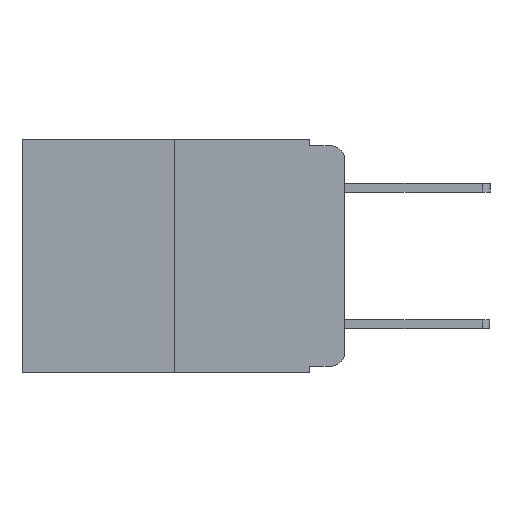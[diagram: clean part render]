
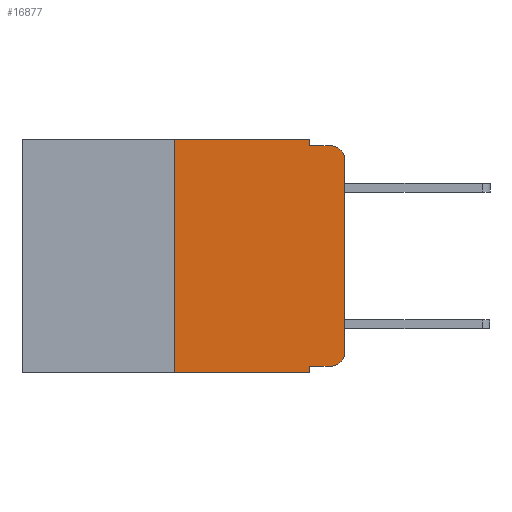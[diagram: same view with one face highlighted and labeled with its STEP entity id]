
A CAD part, left-side view. The second image highlights one B-rep face of the part: STEP entity #16877.
In plain terms, the highlighted planar face has unit normal (-1, 0, 0).
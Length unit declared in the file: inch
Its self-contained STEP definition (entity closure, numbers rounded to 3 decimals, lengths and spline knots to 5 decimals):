
#181 = CARTESIAN_POINT ( 'NONE',  ( 0., 0.02, -0.313 ) ) ;
#188 = ORIENTED_EDGE ( 'NONE', *, *, #11246, .F. ) ;
#422 = VECTOR ( 'NONE', #9994, 39.37008 ) ;
#472 = EDGE_CURVE ( 'NONE', #6923, #17972, #3150, .T. ) ;
#494 = CARTESIAN_POINT ( 'NONE',  ( 0., 0.02, -0.01 ) ) ;
#536 = VECTOR ( 'NONE', #15269, 39.37008 ) ;
#677 = CARTESIAN_POINT ( 'NONE',  ( 0., 0.051, 0. ) ) ;
#696 = DIRECTION ( 'NONE',  ( 0., 0., 1. ) ) ;
#856 = DIRECTION ( 'NONE',  ( 0., 0., -1. ) ) ;
#1072 = ORIENTED_EDGE ( 'NONE', *, *, #9090, .F. ) ;
#1203 = DIRECTION ( 'NONE',  ( 1., 0., 0. ) ) ;
#1535 = EDGE_CURVE ( 'NONE', #9163, #8153, #5222, .T. ) ;
#1844 = DIRECTION ( 'NONE',  ( 0., 0., -1. ) ) ;
#1879 = DIRECTION ( 'NONE',  ( 0., -1., 0. ) ) ;
#1966 = VERTEX_POINT ( 'NONE', #494 ) ;
#2134 = VERTEX_POINT ( 'NONE', #20420 ) ;
#2194 = DIRECTION ( 'NONE',  ( 0., 0., -1. ) ) ;
#2474 = CARTESIAN_POINT ( 'NONE',  ( 0., 0.25, 0. ) ) ;
#3150 = LINE ( 'NONE', #15766, #17242 ) ;
#3175 = CARTESIAN_POINT ( 'NONE',  ( 0., 0., -0.03 ) ) ;
#3643 = VECTOR ( 'NONE', #18622, 39.37008 ) ;
#4335 = EDGE_CURVE ( 'NONE', #6923, #13541, #10631, .T. ) ;
#4337 = VECTOR ( 'NONE', #696, 39.37008 ) ;
#4465 = VERTEX_POINT ( 'NONE', #3175 ) ;
#4986 = CARTESIAN_POINT ( 'NONE',  ( 0., 0.25, 0. ) ) ;
#5062 = CARTESIAN_POINT ( 'NONE',  ( 0., 0., -0.313 ) ) ;
#5222 = LINE ( 'NONE', #677, #20257 ) ;
#5465 = CIRCLE ( 'NONE', #12598, 0.02 ) ;
#5692 = ORIENTED_EDGE ( 'NONE', *, *, #8488, .T. ) ;
#5701 = VECTOR ( 'NONE', #1879, 39.37008 ) ;
#5923 = CARTESIAN_POINT ( 'NONE',  ( 0., 0.051, -0.01 ) ) ;
#6575 = EDGE_LOOP ( 'NONE', ( #7761, #5692, #1072, #21569, #188, #17412, #22151, #22701, #7277, #10739 ) ) ;
#6589 = AXIS2_PLACEMENT_3D ( 'NONE', #12545, #1203, #14337 ) ;
#6639 = CIRCLE ( 'NONE', #22600, 0.02 ) ;
#6923 = VERTEX_POINT ( 'NONE', #18823 ) ;
#7011 = PLANE ( 'NONE',  #6589 ) ;
#7151 = EDGE_CURVE ( 'NONE', #10072, #4465, #23081, .T. ) ;
#7277 = ORIENTED_EDGE ( 'NONE', *, *, #9671, .T. ) ;
#7761 = ORIENTED_EDGE ( 'NONE', *, *, #7151, .T. ) ;
#7845 = CARTESIAN_POINT ( 'NONE',  ( 0., 0.051, -0.333 ) ) ;
#8153 = VERTEX_POINT ( 'NONE', #12173 ) ;
#8488 = EDGE_CURVE ( 'NONE', #4465, #1966, #6639, .T. ) ;
#8598 = EDGE_CURVE ( 'NONE', #2134, #10072, #5465, .T. ) ;
#9090 = EDGE_CURVE ( 'NONE', #8153, #1966, #13510, .T. ) ;
#9163 = VERTEX_POINT ( 'NONE', #17074 ) ;
#9378 = DIRECTION ( 'NONE',  ( 0., -1., 0. ) ) ;
#9511 = CARTESIAN_POINT ( 'NONE',  ( 0., 0.051, -0.333 ) ) ;
#9671 = EDGE_CURVE ( 'NONE', #14532, #2134, #15436, .T. ) ;
#9994 = DIRECTION ( 'NONE',  ( 0., 0., 1. ) ) ;
#10072 = VERTEX_POINT ( 'NONE', #5062 ) ;
#10631 = LINE ( 'NONE', #2474, #422 ) ;
#10739 = ORIENTED_EDGE ( 'NONE', *, *, #8598, .T. ) ;
#11246 = EDGE_CURVE ( 'NONE', #13541, #9163, #15990, .T. ) ;
#12173 = CARTESIAN_POINT ( 'NONE',  ( 0., 0.051, -0.01 ) ) ;
#12250 = CARTESIAN_POINT ( 'NONE',  ( 0., 0., 0. ) ) ;
#12545 = CARTESIAN_POINT ( 'NONE',  ( 0., 0.473, 0. ) ) ;
#12598 = AXIS2_PLACEMENT_3D ( 'NONE', #181, #13422, #2194 ) ;
#13100 = DIRECTION ( 'NONE',  ( -1., 0., 0. ) ) ;
#13422 = DIRECTION ( 'NONE',  ( -1., 0., 0. ) ) ;
#13458 = FACE_OUTER_BOUND ( 'NONE', #6575, .T. ) ;
#13510 = LINE ( 'NONE', #5923, #3643 ) ;
#13541 = VERTEX_POINT ( 'NONE', #4986 ) ;
#14337 = DIRECTION ( 'NONE',  ( 0., 0., -1. ) ) ;
#14532 = VERTEX_POINT ( 'NONE', #7845 ) ;
#15258 = EDGE_CURVE ( 'NONE', #14532, #17972, #20799, .T. ) ;
#15269 = DIRECTION ( 'NONE',  ( 0., 0., -1. ) ) ;
#15436 = LINE ( 'NONE', #9511, #5701 ) ;
#15766 = CARTESIAN_POINT ( 'NONE',  ( 0., 0.473, -0.343 ) ) ;
#15990 = LINE ( 'NONE', #20092, #20161 ) ;
#16877 = ADVANCED_FACE ( 'NONE', ( #13458 ), #7011, .F. ) ;
#17074 = CARTESIAN_POINT ( 'NONE',  ( 0., 0.051, 0. ) ) ;
#17242 = VECTOR ( 'NONE', #23087, 39.37008 ) ;
#17412 = ORIENTED_EDGE ( 'NONE', *, *, #4335, .F. ) ;
#17972 = VERTEX_POINT ( 'NONE', #21226 ) ;
#18622 = DIRECTION ( 'NONE',  ( 0., -1., 0. ) ) ;
#18823 = CARTESIAN_POINT ( 'NONE',  ( 0., 0.25, -0.343 ) ) ;
#20092 = CARTESIAN_POINT ( 'NONE',  ( 0., 0.473, 0. ) ) ;
#20161 = VECTOR ( 'NONE', #9378, 39.37008 ) ;
#20257 = VECTOR ( 'NONE', #856, 39.37008 ) ;
#20420 = CARTESIAN_POINT ( 'NONE',  ( 0., 0.02, -0.333 ) ) ;
#20799 = LINE ( 'NONE', #22348, #536 ) ;
#21226 = CARTESIAN_POINT ( 'NONE',  ( 0., 0.051, -0.343 ) ) ;
#21569 = ORIENTED_EDGE ( 'NONE', *, *, #1535, .F. ) ;
#22151 = ORIENTED_EDGE ( 'NONE', *, *, #472, .T. ) ;
#22348 = CARTESIAN_POINT ( 'NONE',  ( 0., 0.051, 0. ) ) ;
#22600 = AXIS2_PLACEMENT_3D ( 'NONE', #23796, #13100, #1844 ) ;
#22701 = ORIENTED_EDGE ( 'NONE', *, *, #15258, .F. ) ;
#23081 = LINE ( 'NONE', #12250, #4337 ) ;
#23087 = DIRECTION ( 'NONE',  ( 0., -1., 0. ) ) ;
#23796 = CARTESIAN_POINT ( 'NONE',  ( 0., 0.02, -0.03 ) ) ;
